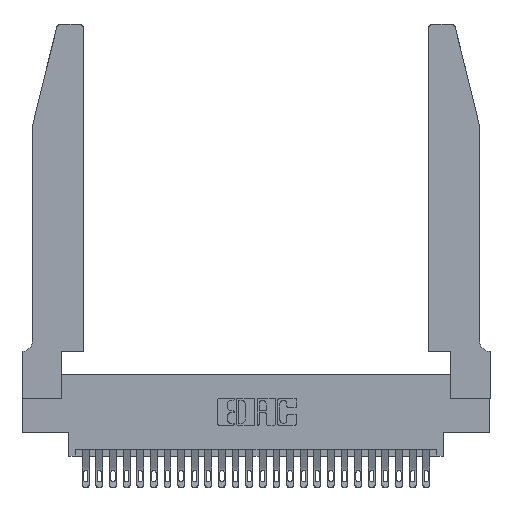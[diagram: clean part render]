
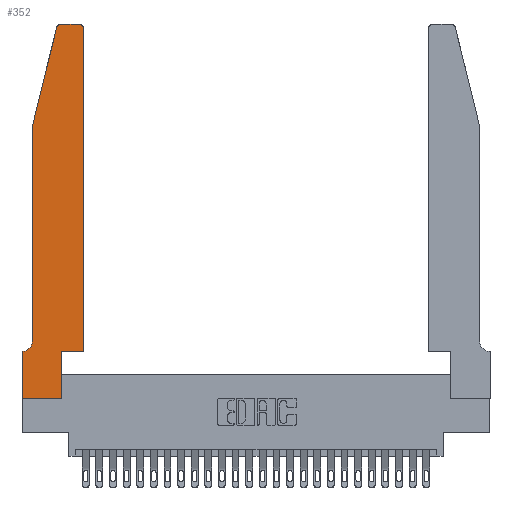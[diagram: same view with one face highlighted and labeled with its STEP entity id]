
A CAD part, top view. The second image highlights one B-rep face of the part: STEP entity #352.
In plain terms, the highlighted planar face has unit normal (0, 0, 1).
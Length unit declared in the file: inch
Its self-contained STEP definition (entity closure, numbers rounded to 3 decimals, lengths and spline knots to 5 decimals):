
#25 = LINE ( 'NONE', #5828, #24188 ) ;
#352 = ADVANCED_FACE ( 'NONE', ( #12144 ), #22709, .T. ) ;
#467 = CARTESIAN_POINT ( 'NONE',  ( 0.0755, 2., 0.37 ) ) ;
#528 = ORIENTED_EDGE ( 'NONE', *, *, #16958, .T. ) ;
#700 = ORIENTED_EDGE ( 'NONE', *, *, #21464, .T. ) ;
#1021 = DIRECTION ( 'NONE',  ( 0., -1., 0. ) ) ;
#1903 = EDGE_CURVE ( 'NONE', #13823, #22768, #9016, .T. ) ;
#2024 = DIRECTION ( 'NONE',  ( 0., 1., 0. ) ) ;
#2406 = VECTOR ( 'NONE', #2024, 39.37008 ) ;
#2701 = CARTESIAN_POINT ( 'NONE',  ( 0.25487, 2.72718, 0.37 ) ) ;
#3014 = DIRECTION ( 'NONE',  ( -1., 0., 0. ) ) ;
#3286 = DIRECTION ( 'NONE',  ( 1., 0., 0. ) ) ;
#3308 = CARTESIAN_POINT ( 'NONE',  ( 0.4205, 2.72, 0.37 ) ) ;
#3326 = CARTESIAN_POINT ( 'NONE',  ( 0.4505, 0.35, 0.37 ) ) ;
#3509 = VECTOR ( 'NONE', #27624, 39.37008 ) ;
#3546 = CARTESIAN_POINT ( 'NONE',  ( 0.4205, 2.75, 0.37 ) ) ;
#4470 = VECTOR ( 'NONE', #3286, 39.37008 ) ;
#4625 = ORIENTED_EDGE ( 'NONE', *, *, #12065, .T. ) ;
#4977 = DIRECTION ( 'NONE',  ( 0., 0., -1. ) ) ;
#5828 = CARTESIAN_POINT ( 'NONE',  ( 0.0755, 0.35, 0.37 ) ) ;
#6503 = VECTOR ( 'NONE', #26236, 39.37008 ) ;
#6560 = VERTEX_POINT ( 'NONE', #9108 ) ;
#6745 = ORIENTED_EDGE ( 'NONE', *, *, #26326, .T. ) ;
#7253 = ORIENTED_EDGE ( 'NONE', *, *, #1903, .T. ) ;
#7280 = CARTESIAN_POINT ( 'NONE',  ( 0.0755, 0.42, 0.37 ) ) ;
#7336 = DIRECTION ( 'NONE',  ( 1., 0., 0. ) ) ;
#7624 = VERTEX_POINT ( 'NONE', #9857 ) ;
#8644 = EDGE_LOOP ( 'NONE', ( #700, #4625, #26416, #6745, #7253, #26843, #18094, #24566, #19770, #15882, #23651, #528 ) ) ;
#9016 = CIRCLE ( 'NONE', #15248, 0.07 ) ;
#9108 = CARTESIAN_POINT ( 'NONE',  ( 0.2865, 0., 0.37 ) ) ;
#9257 = DIRECTION ( 'NONE',  ( 0., -1., 0. ) ) ;
#9612 = CARTESIAN_POINT ( 'NONE',  ( 0.2605, 2.75, 0.37 ) ) ;
#9857 = CARTESIAN_POINT ( 'NONE',  ( 0., 0., 0.37 ) ) ;
#10541 = VECTOR ( 'NONE', #1021, 39.37008 ) ;
#10609 = LINE ( 'NONE', #24328, #14333 ) ;
#11118 = EDGE_CURVE ( 'NONE', #6560, #16100, #15830, .T. ) ;
#11485 = EDGE_CURVE ( 'NONE', #22768, #22719, #25, .T. ) ;
#11665 = CARTESIAN_POINT ( 'NONE',  ( 0., 0.35, 0.37 ) ) ;
#12065 = EDGE_CURVE ( 'NONE', #21013, #25187, #21490, .T. ) ;
#12144 = FACE_OUTER_BOUND ( 'NONE', #8644, .T. ) ;
#12171 = DIRECTION ( 'NONE',  ( 1., 0., 0. ) ) ;
#12634 = VERTEX_POINT ( 'NONE', #3546 ) ;
#12678 = DIRECTION ( 'NONE',  ( 0., 0., 1. ) ) ;
#13823 = VERTEX_POINT ( 'NONE', #7280 ) ;
#14208 = LINE ( 'NONE', #16138, #4470 ) ;
#14333 = VECTOR ( 'NONE', #9257, 39.37008 ) ;
#14354 = DIRECTION ( 'NONE',  ( 0., 0., 1. ) ) ;
#15210 = DIRECTION ( 'NONE',  ( 1., 0., 0. ) ) ;
#15242 = CARTESIAN_POINT ( 'NONE',  ( 0.4505, 2.72, 0.37 ) ) ;
#15248 = AXIS2_PLACEMENT_3D ( 'NONE', #17824, #4977, #19987 ) ;
#15830 = LINE ( 'NONE', #21569, #2406 ) ;
#15866 = CARTESIAN_POINT ( 'NONE',  ( 0.0755, 2., 0.37 ) ) ;
#15882 = ORIENTED_EDGE ( 'NONE', *, *, #24544, .T. ) ;
#16086 = CARTESIAN_POINT ( 'NONE',  ( 0., 0.35, 0.37 ) ) ;
#16100 = VERTEX_POINT ( 'NONE', #17332 ) ;
#16138 = CARTESIAN_POINT ( 'NONE',  ( 0., 0., 0.37 ) ) ;
#16216 = DIRECTION ( 'NONE',  ( 0., 0., 1. ) ) ;
#16958 = EDGE_CURVE ( 'NONE', #23895, #12634, #27555, .T. ) ;
#17239 = CARTESIAN_POINT ( 'NONE',  ( 0.284, 2.72, 0.37 ) ) ;
#17332 = CARTESIAN_POINT ( 'NONE',  ( 0.2865, 0.35, 0.37 ) ) ;
#17824 = CARTESIAN_POINT ( 'NONE',  ( 0.0055, 0.42, 0.37 ) ) ;
#18094 = ORIENTED_EDGE ( 'NONE', *, *, #20497, .T. ) ;
#18318 = CARTESIAN_POINT ( 'NONE',  ( 0.0055, 0.35, 0.37 ) ) ;
#18610 = DIRECTION ( 'NONE',  ( -1., 0., 0. ) ) ;
#18724 = VERTEX_POINT ( 'NONE', #467 ) ;
#19298 = LINE ( 'NONE', #15866, #10541 ) ;
#19473 = VERTEX_POINT ( 'NONE', #3326 ) ;
#19770 = ORIENTED_EDGE ( 'NONE', *, *, #11118, .T. ) ;
#19987 = DIRECTION ( 'NONE',  ( -1., 0., 0. ) ) ;
#20497 = EDGE_CURVE ( 'NONE', #22719, #7624, #10609, .T. ) ;
#20623 = LINE ( 'NONE', #23491, #3509 ) ;
#20959 = AXIS2_PLACEMENT_3D ( 'NONE', #11665, #16216, #7336 ) ;
#21013 = VERTEX_POINT ( 'NONE', #22761 ) ;
#21046 = AXIS2_PLACEMENT_3D ( 'NONE', #3308, #14354, #12171 ) ;
#21464 = EDGE_CURVE ( 'NONE', #12634, #21013, #27393, .T. ) ;
#21490 = CIRCLE ( 'NONE', #24352, 0.03 ) ;
#21566 = DIRECTION ( 'NONE',  ( 1., 0., 0. ) ) ;
#21569 = CARTESIAN_POINT ( 'NONE',  ( 0.2865, 0.35, 0.37 ) ) ;
#21946 = EDGE_CURVE ( 'NONE', #19473, #23895, #27031, .T. ) ;
#21955 = CARTESIAN_POINT ( 'NONE',  ( 0.4505, 0.35, 0.37 ) ) ;
#22208 = VECTOR ( 'NONE', #15210, 39.37008 ) ;
#22246 = EDGE_CURVE ( 'NONE', #25187, #18724, #20623, .T. ) ;
#22709 = PLANE ( 'NONE',  #20959 ) ;
#22719 = VERTEX_POINT ( 'NONE', #16086 ) ;
#22761 = CARTESIAN_POINT ( 'NONE',  ( 0.284, 2.75, 0.37 ) ) ;
#22768 = VERTEX_POINT ( 'NONE', #18318 ) ;
#23237 = EDGE_CURVE ( 'NONE', #7624, #6560, #14208, .T. ) ;
#23491 = CARTESIAN_POINT ( 'NONE',  ( 0.0755, 2., 0.37 ) ) ;
#23651 = ORIENTED_EDGE ( 'NONE', *, *, #21946, .T. ) ;
#23706 = VECTOR ( 'NONE', #3014, 39.37008 ) ;
#23895 = VERTEX_POINT ( 'NONE', #15242 ) ;
#24188 = VECTOR ( 'NONE', #18610, 39.37008 ) ;
#24328 = CARTESIAN_POINT ( 'NONE',  ( 0., 0., 0.37 ) ) ;
#24352 = AXIS2_PLACEMENT_3D ( 'NONE', #17239, #12678, #21566 ) ;
#24544 = EDGE_CURVE ( 'NONE', #16100, #19473, #26891, .T. ) ;
#24566 = ORIENTED_EDGE ( 'NONE', *, *, #23237, .T. ) ;
#25187 = VERTEX_POINT ( 'NONE', #2701 ) ;
#25873 = CARTESIAN_POINT ( 'NONE',  ( 0.4505, 0.35, 0.37 ) ) ;
#26236 = DIRECTION ( 'NONE',  ( 0., 1., 0. ) ) ;
#26326 = EDGE_CURVE ( 'NONE', #18724, #13823, #19298, .T. ) ;
#26416 = ORIENTED_EDGE ( 'NONE', *, *, #22246, .T. ) ;
#26843 = ORIENTED_EDGE ( 'NONE', *, *, #11485, .T. ) ;
#26891 = LINE ( 'NONE', #25873, #22208 ) ;
#27031 = LINE ( 'NONE', #21955, #6503 ) ;
#27393 = LINE ( 'NONE', #9612, #23706 ) ;
#27555 = CIRCLE ( 'NONE', #21046, 0.03 ) ;
#27624 = DIRECTION ( 'NONE',  ( -0.239, -0.971, 0. ) ) ;
